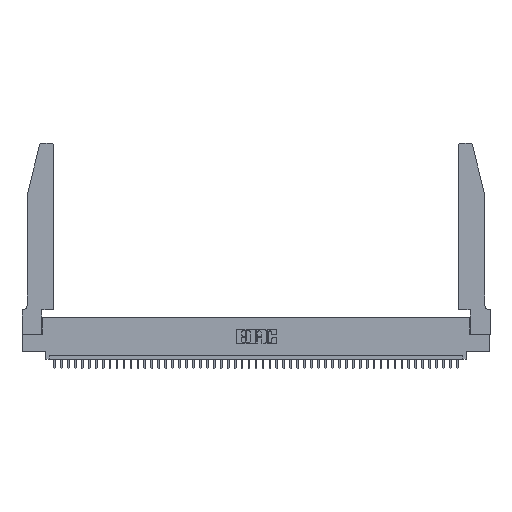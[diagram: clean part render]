
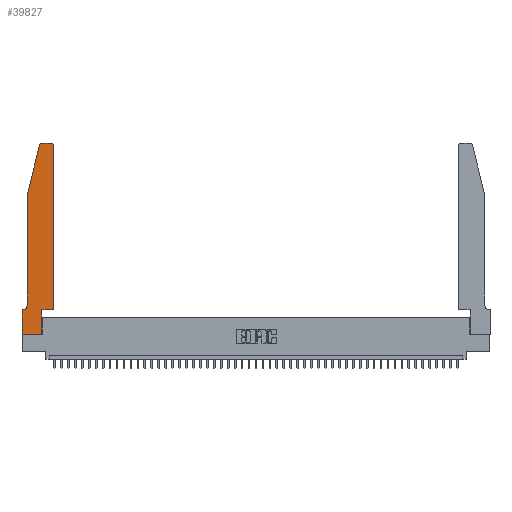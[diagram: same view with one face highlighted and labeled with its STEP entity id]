
A CAD part, top view. The second image highlights one B-rep face of the part: STEP entity #39827.
In plain terms, the highlighted planar face has unit normal (0, 0, 1).
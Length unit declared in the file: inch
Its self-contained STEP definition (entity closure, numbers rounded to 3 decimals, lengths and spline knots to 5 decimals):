
#1993 = EDGE_CURVE ( 'NONE', #18045, #13505, #11310, .T. ) ;
#2681 = ORIENTED_EDGE ( 'NONE', *, *, #5579, .T. ) ;
#2949 = VECTOR ( 'NONE', #24091, 39.37008 ) ;
#4734 = CARTESIAN_POINT ( 'NONE',  ( 0., 0., 0.37 ) ) ;
#5405 = AXIS2_PLACEMENT_3D ( 'NONE', #20552, #46017, #24202 ) ;
#5579 = EDGE_CURVE ( 'NONE', #19778, #39801, #24074, .T. ) ;
#5810 = VECTOR ( 'NONE', #34118, 39.37008 ) ;
#7140 = CARTESIAN_POINT ( 'NONE',  ( 0.284, 2.75, 0.37 ) ) ;
#7310 = EDGE_LOOP ( 'NONE', ( #29842, #43729, #42230, #29580, #2681, #29717, #20506, #35602, #39636, #45030, #15310, #40854 ) ) ;
#8428 = VECTOR ( 'NONE', #19866, 39.37008 ) ;
#8944 = VERTEX_POINT ( 'NONE', #7140 ) ;
#9210 = EDGE_CURVE ( 'NONE', #13505, #34708, #24545, .T. ) ;
#9598 = EDGE_CURVE ( 'NONE', #18182, #22394, #28444, .T. ) ;
#10002 = CARTESIAN_POINT ( 'NONE',  ( 0.4505, 2.72, 0.37 ) ) ;
#10306 = DIRECTION ( 'NONE',  ( 1., 0., 0. ) ) ;
#10984 = EDGE_CURVE ( 'NONE', #39801, #14745, #45901, .T. ) ;
#11310 = LINE ( 'NONE', #19692, #8428 ) ;
#11552 = LINE ( 'NONE', #26563, #38969 ) ;
#12932 = VECTOR ( 'NONE', #33363, 39.37008 ) ;
#13438 = EDGE_CURVE ( 'NONE', #33517, #26840, #11552, .T. ) ;
#13505 = VERTEX_POINT ( 'NONE', #36319 ) ;
#13722 = LINE ( 'NONE', #45581, #2949 ) ;
#13787 = CIRCLE ( 'NONE', #40237, 0.03 ) ;
#14672 = VECTOR ( 'NONE', #37657, 39.37008 ) ;
#14745 = VERTEX_POINT ( 'NONE', #23184 ) ;
#15310 = ORIENTED_EDGE ( 'NONE', *, *, #9210, .T. ) ;
#15575 = DIRECTION ( 'NONE',  ( -1., 0., 0. ) ) ;
#17238 = DIRECTION ( 'NONE',  ( 0., 0., 1. ) ) ;
#18045 = VERTEX_POINT ( 'NONE', #30577 ) ;
#18182 = VERTEX_POINT ( 'NONE', #28378 ) ;
#18398 = CARTESIAN_POINT ( 'NONE',  ( 0., 0.35, 0.37 ) ) ;
#19213 = CARTESIAN_POINT ( 'NONE',  ( 0.0755, 0.42, 0.37 ) ) ;
#19692 = CARTESIAN_POINT ( 'NONE',  ( 0.4505, 0.35, 0.37 ) ) ;
#19778 = VERTEX_POINT ( 'NONE', #19213 ) ;
#19866 = DIRECTION ( 'NONE',  ( 1., 0., 0. ) ) ;
#20128 = EDGE_CURVE ( 'NONE', #8944, #33517, #13787, .T. ) ;
#20506 = ORIENTED_EDGE ( 'NONE', *, *, #25634, .T. ) ;
#20552 = CARTESIAN_POINT ( 'NONE',  ( 0.0055, 0.42, 0.37 ) ) ;
#21294 = CIRCLE ( 'NONE', #37129, 0.03 ) ;
#21373 = LINE ( 'NONE', #40606, #39647 ) ;
#22354 = VERTEX_POINT ( 'NONE', #24470 ) ;
#22394 = VERTEX_POINT ( 'NONE', #31624 ) ;
#23184 = CARTESIAN_POINT ( 'NONE',  ( 0., 0.35, 0.37 ) ) ;
#23541 = AXIS2_PLACEMENT_3D ( 'NONE', #18398, #43856, #32993 ) ;
#24074 = CIRCLE ( 'NONE', #5405, 0.07 ) ;
#24091 = DIRECTION ( 'NONE',  ( 0., 1., 0. ) ) ;
#24202 = DIRECTION ( 'NONE',  ( -1., 0., 0. ) ) ;
#24470 = CARTESIAN_POINT ( 'NONE',  ( 0.4205, 2.75, 0.37 ) ) ;
#24545 = LINE ( 'NONE', #32784, #5810 ) ;
#24850 = CARTESIAN_POINT ( 'NONE',  ( 0.284, 2.72, 0.37 ) ) ;
#25542 = PLANE ( 'NONE',  #23541 ) ;
#25634 = EDGE_CURVE ( 'NONE', #14745, #18182, #25845, .T. ) ;
#25845 = LINE ( 'NONE', #4734, #36136 ) ;
#26563 = CARTESIAN_POINT ( 'NONE',  ( 0.0755, 2., 0.37 ) ) ;
#26840 = VERTEX_POINT ( 'NONE', #30866 ) ;
#27051 = FACE_OUTER_BOUND ( 'NONE', #7310, .T. ) ;
#28378 = CARTESIAN_POINT ( 'NONE',  ( 0., 0., 0.37 ) ) ;
#28444 = LINE ( 'NONE', #42052, #46698 ) ;
#28882 = CARTESIAN_POINT ( 'NONE',  ( 0.0055, 0.35, 0.37 ) ) ;
#29580 = ORIENTED_EDGE ( 'NONE', *, *, #39359, .T. ) ;
#29717 = ORIENTED_EDGE ( 'NONE', *, *, #10984, .T. ) ;
#29842 = ORIENTED_EDGE ( 'NONE', *, *, #40547, .T. ) ;
#30254 = DIRECTION ( 'NONE',  ( 0., -1., 0. ) ) ;
#30451 = DIRECTION ( 'NONE',  ( 1., 0., 0. ) ) ;
#30577 = CARTESIAN_POINT ( 'NONE',  ( 0.2865, 0.35, 0.37 ) ) ;
#30866 = CARTESIAN_POINT ( 'NONE',  ( 0.0755, 2., 0.37 ) ) ;
#31384 = CARTESIAN_POINT ( 'NONE',  ( 0.0755, 0.35, 0.37 ) ) ;
#31624 = CARTESIAN_POINT ( 'NONE',  ( 0.2865, 0., 0.37 ) ) ;
#32784 = CARTESIAN_POINT ( 'NONE',  ( 0.4505, 0.35, 0.37 ) ) ;
#32993 = DIRECTION ( 'NONE',  ( 1., 0., 0. ) ) ;
#33363 = DIRECTION ( 'NONE',  ( -1., 0., 0. ) ) ;
#33517 = VERTEX_POINT ( 'NONE', #39360 ) ;
#33920 = EDGE_CURVE ( 'NONE', #34708, #22354, #21294, .T. ) ;
#34118 = DIRECTION ( 'NONE',  ( 0., 1., 0. ) ) ;
#34302 = CARTESIAN_POINT ( 'NONE',  ( 0.0755, 2., 0.37 ) ) ;
#34708 = VERTEX_POINT ( 'NONE', #10002 ) ;
#35602 = ORIENTED_EDGE ( 'NONE', *, *, #9598, .T. ) ;
#36136 = VECTOR ( 'NONE', #30254, 39.37008 ) ;
#36319 = CARTESIAN_POINT ( 'NONE',  ( 0.4505, 0.35, 0.37 ) ) ;
#37129 = AXIS2_PLACEMENT_3D ( 'NONE', #37635, #44792, #30451 ) ;
#37635 = CARTESIAN_POINT ( 'NONE',  ( 0.4205, 2.72, 0.37 ) ) ;
#37657 = DIRECTION ( 'NONE',  ( 0., -1., 0. ) ) ;
#38969 = VECTOR ( 'NONE', #42098, 39.37008 ) ;
#39359 = EDGE_CURVE ( 'NONE', #26840, #19778, #44798, .T. ) ;
#39360 = CARTESIAN_POINT ( 'NONE',  ( 0.25487, 2.72718, 0.37 ) ) ;
#39636 = ORIENTED_EDGE ( 'NONE', *, *, #44372, .T. ) ;
#39647 = VECTOR ( 'NONE', #15575, 39.37008 ) ;
#39801 = VERTEX_POINT ( 'NONE', #28882 ) ;
#39827 = ADVANCED_FACE ( 'NONE', ( #27051 ), #25542, .T. ) ;
#40237 = AXIS2_PLACEMENT_3D ( 'NONE', #24850, #17238, #10306 ) ;
#40547 = EDGE_CURVE ( 'NONE', #22354, #8944, #21373, .T. ) ;
#40606 = CARTESIAN_POINT ( 'NONE',  ( 0.2605, 2.75, 0.37 ) ) ;
#40854 = ORIENTED_EDGE ( 'NONE', *, *, #33920, .T. ) ;
#42052 = CARTESIAN_POINT ( 'NONE',  ( 0., 0., 0.37 ) ) ;
#42098 = DIRECTION ( 'NONE',  ( -0.239, -0.971, 0. ) ) ;
#42230 = ORIENTED_EDGE ( 'NONE', *, *, #13438, .T. ) ;
#42374 = DIRECTION ( 'NONE',  ( 1., 0., 0. ) ) ;
#43729 = ORIENTED_EDGE ( 'NONE', *, *, #20128, .T. ) ;
#43856 = DIRECTION ( 'NONE',  ( 0., 0., 1. ) ) ;
#44372 = EDGE_CURVE ( 'NONE', #22394, #18045, #13722, .T. ) ;
#44792 = DIRECTION ( 'NONE',  ( 0., 0., 1. ) ) ;
#44798 = LINE ( 'NONE', #34302, #14672 ) ;
#45030 = ORIENTED_EDGE ( 'NONE', *, *, #1993, .T. ) ;
#45581 = CARTESIAN_POINT ( 'NONE',  ( 0.2865, 0.35, 0.37 ) ) ;
#45901 = LINE ( 'NONE', #31384, #12932 ) ;
#46017 = DIRECTION ( 'NONE',  ( 0., 0., -1. ) ) ;
#46698 = VECTOR ( 'NONE', #42374, 39.37008 ) ;
